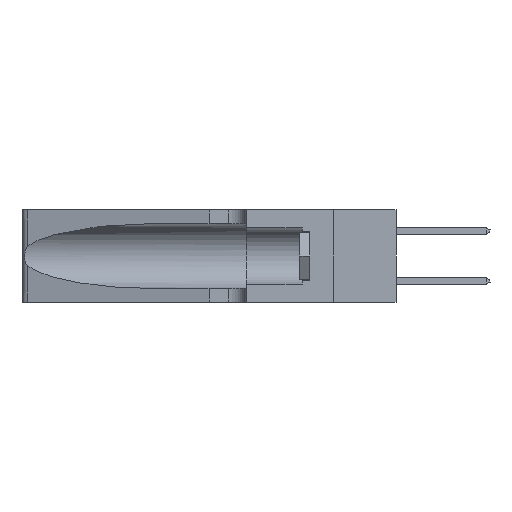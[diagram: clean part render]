
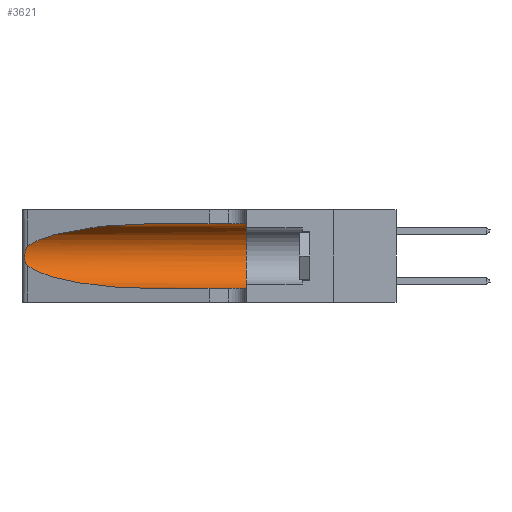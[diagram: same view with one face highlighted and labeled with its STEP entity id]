
A CAD part, left-side view. The second image highlights one B-rep face of the part: STEP entity #3621.
In plain terms, the highlighted cylindrical face has radius 3.308 mm (diameter 6.617 mm), a partial arc.
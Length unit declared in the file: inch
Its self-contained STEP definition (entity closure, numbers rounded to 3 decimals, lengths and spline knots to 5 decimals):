
#112 = B_SPLINE_CURVE_WITH_KNOTS ( 'NONE', 3,
 ( #18975, #24804, #13261, #1385, #15190, #3417, #17133, #5425, #19061, #7451, #21020, #9426, #22961, #11395 ),
 .UNSPECIFIED., .F., .F.,
 ( 4, 2, 2, 2, 2, 2, 4 ),
 ( 0., 0.00027, 0.00053, 0.00107, 0.0016, 0.00187, 0.00214 ),
 .UNSPECIFIED. ) ;
#145 = EDGE_CURVE ( 'NONE', #19817, #4401, #2087, .T. ) ;
#329 = CARTESIAN_POINT ( 'NONE',  ( 0.1305, 0.72297, 0.31525 ) ) ;
#568 = DIRECTION ( 'NONE',  ( 0., 0., -1. ) ) ;
#1192 = EDGE_CURVE ( 'NONE', #20163, #15581, #11839, .T. ) ;
#1385 = CARTESIAN_POINT ( 'NONE',  ( 0.25787, 1.23484, 0.2124 ) ) ;
#2048 = ORIENTED_EDGE ( 'NONE', *, *, #5192, .T. ) ;
#2087 =( BOUNDED_CURVE ( )  B_SPLINE_CURVE ( 3, ( #8694, #7877, #11925, #11892 ),
 .UNSPECIFIED., .F., .F. ) 
 B_SPLINE_CURVE_WITH_KNOTS ( ( 4, 4 ),
 ( 3.44316, 4.71239 ),
 .UNSPECIFIED. ) 
 CURVE ( )  GEOMETRIC_REPRESENTATION_ITEM ( )  RATIONAL_B_SPLINE_CURVE ( ( 1., 0.87, 0.87, 1. ) ) 
 REPRESENTATION_ITEM ( '' )  );
#2238 = CIRCLE ( 'NONE', #5658, 0.13025 ) ;
#2326 = CARTESIAN_POINT ( 'NONE',  ( 0.1305, 1.61858, 0.05475 ) ) ;
#2992 = VERTEX_POINT ( 'NONE', #8511 ) ;
#3370 = CARTESIAN_POINT ( 'NONE',  ( 0.25487, 1.22718, 0.22369 ) ) ;
#3417 = CARTESIAN_POINT ( 'NONE',  ( 0.26018, 1.23835, 0.19895 ) ) ;
#3621 = ADVANCED_FACE ( 'NONE', ( #8742 ), #8134, .F. ) ;
#4401 = VERTEX_POINT ( 'NONE', #20552 ) ;
#4538 = EDGE_CURVE ( 'NONE', #20163, #2992, #13972, .T. ) ;
#4668 = DIRECTION ( 'NONE',  ( 0., -1., 0. ) ) ;
#5192 = EDGE_CURVE ( 'NONE', #4401, #17588, #10188, .T. ) ;
#5425 = CARTESIAN_POINT ( 'NONE',  ( 0.26075, 1.23896, 0.178 ) ) ;
#5658 = AXIS2_PLACEMENT_3D ( 'NONE', #6832, #20401, #8808 ) ;
#5690 = ORIENTED_EDGE ( 'NONE', *, *, #4538, .T. ) ;
#6766 = CARTESIAN_POINT ( 'NONE',  ( 0.1305, 1.61858, 0.31525 ) ) ;
#6832 = CARTESIAN_POINT ( 'NONE',  ( 0.1305, 0.35, 0.185 ) ) ;
#7451 = CARTESIAN_POINT ( 'NONE',  ( 0.25856, 1.23593, 0.16098 ) ) ;
#7877 = CARTESIAN_POINT ( 'NONE',  ( 0.2373, 1.15595, 0.08982 ) ) ;
#8134 = CYLINDRICAL_SURFACE ( 'NONE', #24458, 0.13025 ) ;
#8452 = ORIENTED_EDGE ( 'NONE', *, *, #145, .T. ) ;
#8511 = CARTESIAN_POINT ( 'NONE',  ( 0.25487, 1.22718, 0.22369 ) ) ;
#8630 = ORIENTED_EDGE ( 'NONE', *, *, #1192, .F. ) ;
#8694 = CARTESIAN_POINT ( 'NONE',  ( 0.25487, 1.22718, 0.14631 ) ) ;
#8742 = FACE_OUTER_BOUND ( 'NONE', #14366, .T. ) ;
#8808 = DIRECTION ( 'NONE',  ( 0., 0., 1. ) ) ;
#9387 = EDGE_CURVE ( 'NONE', #15581, #17588, #2238, .T. ) ;
#9426 = CARTESIAN_POINT ( 'NONE',  ( 0.25639, 1.23186, 0.15144 ) ) ;
#10188 = LINE ( 'NONE', #2326, #19867 ) ;
#10991 = CARTESIAN_POINT ( 'NONE',  ( 0.1305, 0.35, 0.31525 ) ) ;
#11395 = CARTESIAN_POINT ( 'NONE',  ( 0.25487, 1.22718, 0.14631 ) ) ;
#11839 = LINE ( 'NONE', #6766, #21507 ) ;
#11892 = CARTESIAN_POINT ( 'NONE',  ( 0.1305, 0.72297, 0.05475 ) ) ;
#11925 = CARTESIAN_POINT ( 'NONE',  ( 0.18966, 0.96281, 0.05475 ) ) ;
#12108 = EDGE_CURVE ( 'NONE', #2992, #19817, #112, .T. ) ;
#13261 = CARTESIAN_POINT ( 'NONE',  ( 0.25639, 1.23184, 0.21858 ) ) ;
#13972 =( BOUNDED_CURVE ( )  B_SPLINE_CURVE ( 3, ( #18932, #22835, #15143, #3370 ),
 .UNSPECIFIED., .F., .F. ) 
 B_SPLINE_CURVE_WITH_KNOTS ( ( 4, 4 ),
 ( 1.5708, 2.84003 ),
 .UNSPECIFIED. ) 
 CURVE ( )  GEOMETRIC_REPRESENTATION_ITEM ( )  RATIONAL_B_SPLINE_CURVE ( ( 1., 0.87, 0.87, 1. ) ) 
 REPRESENTATION_ITEM ( '' )  );
#14153 = DIRECTION ( 'NONE',  ( 0., -1., 0. ) ) ;
#14366 = EDGE_LOOP ( 'NONE', ( #5690, #19638, #8452, #2048, #16158, #8630 ) ) ;
#15143 = CARTESIAN_POINT ( 'NONE',  ( 0.2373, 1.15595, 0.28018 ) ) ;
#15190 = CARTESIAN_POINT ( 'NONE',  ( 0.25854, 1.2359, 0.20912 ) ) ;
#15581 = VERTEX_POINT ( 'NONE', #10991 ) ;
#16158 = ORIENTED_EDGE ( 'NONE', *, *, #9387, .F. ) ;
#16450 = CARTESIAN_POINT ( 'NONE',  ( 0.1305, 0.35, 0.05475 ) ) ;
#17133 = CARTESIAN_POINT ( 'NONE',  ( 0.26075, 1.23896, 0.19203 ) ) ;
#17588 = VERTEX_POINT ( 'NONE', #16450 ) ;
#18303 = DIRECTION ( 'NONE',  ( 0., -1., 0. ) ) ;
#18932 = CARTESIAN_POINT ( 'NONE',  ( 0.1305, 0.72297, 0.31525 ) ) ;
#18975 = CARTESIAN_POINT ( 'NONE',  ( 0.25487, 1.22718, 0.22369 ) ) ;
#19061 = CARTESIAN_POINT ( 'NONE',  ( 0.26017, 1.23833, 0.17102 ) ) ;
#19638 = ORIENTED_EDGE ( 'NONE', *, *, #12108, .T. ) ;
#19817 = VERTEX_POINT ( 'NONE', #25206 ) ;
#19867 = VECTOR ( 'NONE', #14153, 39.37008 ) ;
#20163 = VERTEX_POINT ( 'NONE', #329 ) ;
#20237 = CARTESIAN_POINT ( 'NONE',  ( 0.1305, 1.61858, 0.185 ) ) ;
#20401 = DIRECTION ( 'NONE',  ( 0., 1., 0. ) ) ;
#20552 = CARTESIAN_POINT ( 'NONE',  ( 0.1305, 0.72297, 0.05475 ) ) ;
#21020 = CARTESIAN_POINT ( 'NONE',  ( 0.25789, 1.23486, 0.15765 ) ) ;
#21507 = VECTOR ( 'NONE', #4668, 39.37008 ) ;
#22835 = CARTESIAN_POINT ( 'NONE',  ( 0.18966, 0.96281, 0.31525 ) ) ;
#22961 = CARTESIAN_POINT ( 'NONE',  ( 0.25555, 1.22993, 0.14849 ) ) ;
#24458 = AXIS2_PLACEMENT_3D ( 'NONE', #20237, #18303, #568 ) ;
#24804 = CARTESIAN_POINT ( 'NONE',  ( 0.25555, 1.22994, 0.2215 ) ) ;
#25206 = CARTESIAN_POINT ( 'NONE',  ( 0.25487, 1.22718, 0.14631 ) ) ;
